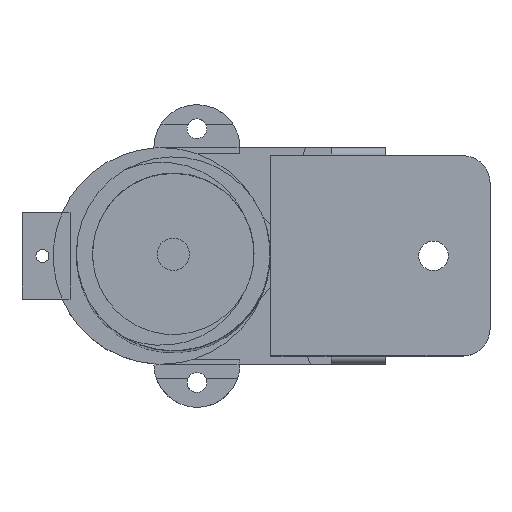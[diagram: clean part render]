
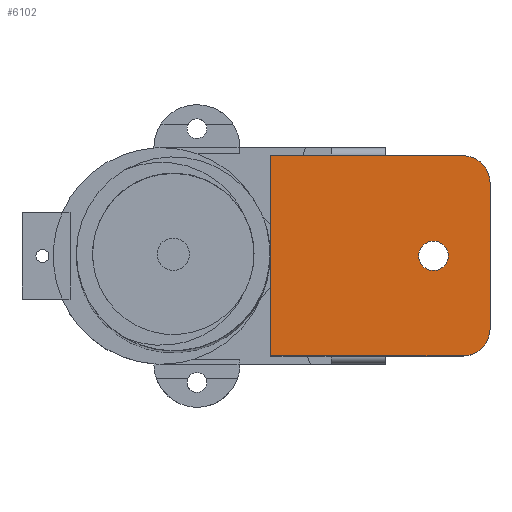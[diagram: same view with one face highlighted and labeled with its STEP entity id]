
A CAD part, top view. The second image highlights one B-rep face of the part: STEP entity #6102.
In plain terms, the highlighted planar face has unit normal (0, 0, 1).
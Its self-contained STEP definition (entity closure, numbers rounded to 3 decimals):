
#3898 = PLANE('',#3899);
#3899 = AXIS2_PLACEMENT_3D('',#3900,#3901,#3902);
#3900 = CARTESIAN_POINT('',(-27.612,18.6,22.6));
#3901 = DIRECTION('',(0.,1.,0.));
#3902 = DIRECTION('',(1.,0.,0.));
#4639 = PLANE('',#4640);
#4640 = AXIS2_PLACEMENT_3D('',#4641,#4642,#4643);
#4641 = CARTESIAN_POINT('',(13.137,-18.6,22.6));
#4642 = DIRECTION('',(0.,-1.,0.));
#4643 = DIRECTION('',(-1.,0.,0.));
#5168 = PLANE('',#5169);
#5169 = AXIS2_PLACEMENT_3D('',#5170,#5171,#5172);
#5170 = CARTESIAN_POINT('',(-27.612,-18.6,22.6));
#5171 = DIRECTION('',(-1.,0.,0.));
#5172 = DIRECTION('',(0.,1.,0.));
#5205 = EDGE_CURVE('',#5206,#5208,#5210,.T.);
#5206 = VERTEX_POINT('',#5207);
#5207 = CARTESIAN_POINT('',(-27.612,18.6,24.1));
#5208 = VERTEX_POINT('',#5209);
#5209 = CARTESIAN_POINT('',(8.137,18.6,24.1));
#5210 = SURFACE_CURVE('',#5211,(#5215,#5222),.PCURVE_S1.);
#5211 = LINE('',#5212,#5213);
#5212 = CARTESIAN_POINT('',(-27.612,18.6,24.1));
#5213 = VECTOR('',#5214,1.);
#5214 = DIRECTION('',(1.,0.,0.));
#5215 = PCURVE('',#3898,#5216);
#5216 = DEFINITIONAL_REPRESENTATION('',(#5217),#5221);
#5217 = LINE('',#5218,#5219);
#5218 = CARTESIAN_POINT('',(0.,-1.5));
#5219 = VECTOR('',#5220,1.);
#5220 = DIRECTION('',(1.,0.));
#5221 = ( GEOMETRIC_REPRESENTATION_CONTEXT(2) 
PARAMETRIC_REPRESENTATION_CONTEXT() REPRESENTATION_CONTEXT('2D SPACE',''
  ) );
#5222 = PCURVE('',#5223,#5228);
#5223 = PLANE('',#5224);
#5224 = AXIS2_PLACEMENT_3D('',#5225,#5226,#5227);
#5225 = CARTESIAN_POINT('',(-27.612,18.6,24.1));
#5226 = DIRECTION('',(0.,0.,1.));
#5227 = DIRECTION('',(1.,0.,0.));
#5228 = DEFINITIONAL_REPRESENTATION('',(#5229),#5233);
#5229 = LINE('',#5230,#5231);
#5230 = CARTESIAN_POINT('',(0.,0.));
#5231 = VECTOR('',#5232,1.);
#5232 = DIRECTION('',(1.,0.));
#5233 = ( GEOMETRIC_REPRESENTATION_CONTEXT(2) 
PARAMETRIC_REPRESENTATION_CONTEXT() REPRESENTATION_CONTEXT('2D SPACE',''
  ) );
#5251 = CYLINDRICAL_SURFACE('',#5252,5.);
#5252 = AXIS2_PLACEMENT_3D('',#5253,#5254,#5255);
#5253 = CARTESIAN_POINT('',(8.137,13.6,22.6));
#5254 = DIRECTION('',(0.,0.,1.));
#5255 = DIRECTION('',(1.,0.,0.));
#5709 = EDGE_CURVE('',#5710,#5712,#5714,.T.);
#5710 = VERTEX_POINT('',#5711);
#5711 = CARTESIAN_POINT('',(8.137,-18.6,24.1));
#5712 = VERTEX_POINT('',#5713);
#5713 = CARTESIAN_POINT('',(-27.612,-18.6,24.1));
#5714 = SURFACE_CURVE('',#5715,(#5719,#5726),.PCURVE_S1.);
#5715 = LINE('',#5716,#5717);
#5716 = CARTESIAN_POINT('',(13.137,-18.6,24.1));
#5717 = VECTOR('',#5718,1.);
#5718 = DIRECTION('',(-1.,0.,0.));
#5719 = PCURVE('',#4639,#5720);
#5720 = DEFINITIONAL_REPRESENTATION('',(#5721),#5725);
#5721 = LINE('',#5722,#5723);
#5722 = CARTESIAN_POINT('',(0.,-1.5));
#5723 = VECTOR('',#5724,1.);
#5724 = DIRECTION('',(1.,0.));
#5725 = ( GEOMETRIC_REPRESENTATION_CONTEXT(2) 
PARAMETRIC_REPRESENTATION_CONTEXT() REPRESENTATION_CONTEXT('2D SPACE',''
  ) );
#5726 = PCURVE('',#5223,#5727);
#5727 = DEFINITIONAL_REPRESENTATION('',(#5728),#5732);
#5728 = LINE('',#5729,#5730);
#5729 = CARTESIAN_POINT('',(40.749,-37.2));
#5730 = VECTOR('',#5731,1.);
#5731 = DIRECTION('',(-1.,0.));
#5732 = ( GEOMETRIC_REPRESENTATION_CONTEXT(2) 
PARAMETRIC_REPRESENTATION_CONTEXT() REPRESENTATION_CONTEXT('2D SPACE',''
  ) );
#5795 = CYLINDRICAL_SURFACE('',#5796,5.);
#5796 = AXIS2_PLACEMENT_3D('',#5797,#5798,#5799);
#5797 = CARTESIAN_POINT('',(8.137,-13.6,22.6));
#5798 = DIRECTION('',(0.,0.,1.));
#5799 = DIRECTION('',(1.,0.,0.));
#6080 = EDGE_CURVE('',#5712,#5206,#6081,.T.);
#6081 = SURFACE_CURVE('',#6082,(#6086,#6093),.PCURVE_S1.);
#6082 = LINE('',#6083,#6084);
#6083 = CARTESIAN_POINT('',(-27.612,-18.6,24.1));
#6084 = VECTOR('',#6085,1.);
#6085 = DIRECTION('',(0.,1.,0.));
#6086 = PCURVE('',#5168,#6087);
#6087 = DEFINITIONAL_REPRESENTATION('',(#6088),#6092);
#6088 = LINE('',#6089,#6090);
#6089 = CARTESIAN_POINT('',(0.,-1.5));
#6090 = VECTOR('',#6091,1.);
#6091 = DIRECTION('',(1.,0.));
#6092 = ( GEOMETRIC_REPRESENTATION_CONTEXT(2) 
PARAMETRIC_REPRESENTATION_CONTEXT() REPRESENTATION_CONTEXT('2D SPACE',''
  ) );
#6093 = PCURVE('',#5223,#6094);
#6094 = DEFINITIONAL_REPRESENTATION('',(#6095),#6099);
#6095 = LINE('',#6096,#6097);
#6096 = CARTESIAN_POINT('',(0.,-37.2));
#6097 = VECTOR('',#6098,1.);
#6098 = DIRECTION('',(0.,1.));
#6099 = ( GEOMETRIC_REPRESENTATION_CONTEXT(2) 
PARAMETRIC_REPRESENTATION_CONTEXT() REPRESENTATION_CONTEXT('2D SPACE',''
  ) );
#6102 = ADVANCED_FACE('',(#6103,#6186),#5223,.T.);
#6103 = FACE_BOUND('',#6104,.T.);
#6104 = EDGE_LOOP('',(#6105,#6135,#6157,#6158,#6159,#6160));
#6105 = ORIENTED_EDGE('',*,*,#6106,.F.);
#6106 = EDGE_CURVE('',#6107,#6109,#6111,.T.);
#6107 = VERTEX_POINT('',#6108);
#6108 = CARTESIAN_POINT('',(13.137,13.6,24.1));
#6109 = VERTEX_POINT('',#6110);
#6110 = CARTESIAN_POINT('',(13.137,-13.6,24.1));
#6111 = SURFACE_CURVE('',#6112,(#6116,#6123),.PCURVE_S1.);
#6112 = LINE('',#6113,#6114);
#6113 = CARTESIAN_POINT('',(13.137,18.6,24.1));
#6114 = VECTOR('',#6115,1.);
#6115 = DIRECTION('',(0.,-1.,0.));
#6116 = PCURVE('',#5223,#6117);
#6117 = DEFINITIONAL_REPRESENTATION('',(#6118),#6122);
#6118 = LINE('',#6119,#6120);
#6119 = CARTESIAN_POINT('',(40.749,0.));
#6120 = VECTOR('',#6121,1.);
#6121 = DIRECTION('',(0.,-1.));
#6122 = ( GEOMETRIC_REPRESENTATION_CONTEXT(2) 
PARAMETRIC_REPRESENTATION_CONTEXT() REPRESENTATION_CONTEXT('2D SPACE',''
  ) );
#6123 = PCURVE('',#6124,#6129);
#6124 = PLANE('',#6125);
#6125 = AXIS2_PLACEMENT_3D('',#6126,#6127,#6128);
#6126 = CARTESIAN_POINT('',(13.137,18.6,22.6));
#6127 = DIRECTION('',(1.,0.,0.));
#6128 = DIRECTION('',(0.,-1.,0.));
#6129 = DEFINITIONAL_REPRESENTATION('',(#6130),#6134);
#6130 = LINE('',#6131,#6132);
#6131 = CARTESIAN_POINT('',(0.,-1.5));
#6132 = VECTOR('',#6133,1.);
#6133 = DIRECTION('',(1.,0.));
#6134 = ( GEOMETRIC_REPRESENTATION_CONTEXT(2) 
PARAMETRIC_REPRESENTATION_CONTEXT() REPRESENTATION_CONTEXT('2D SPACE',''
  ) );
#6135 = ORIENTED_EDGE('',*,*,#6136,.T.);
#6136 = EDGE_CURVE('',#6107,#5208,#6137,.T.);
#6137 = SURFACE_CURVE('',#6138,(#6143,#6150),.PCURVE_S1.);
#6138 = CIRCLE('',#6139,5.);
#6139 = AXIS2_PLACEMENT_3D('',#6140,#6141,#6142);
#6140 = CARTESIAN_POINT('',(8.137,13.6,24.1));
#6141 = DIRECTION('',(0.,0.,1.));
#6142 = DIRECTION('',(0.,-1.,0.));
#6143 = PCURVE('',#5223,#6144);
#6144 = DEFINITIONAL_REPRESENTATION('',(#6145),#6149);
#6145 = CIRCLE('',#6146,5.);
#6146 = AXIS2_PLACEMENT_2D('',#6147,#6148);
#6147 = CARTESIAN_POINT('',(35.749,-5.));
#6148 = DIRECTION('',(0.,-1.));
#6149 = ( GEOMETRIC_REPRESENTATION_CONTEXT(2) 
PARAMETRIC_REPRESENTATION_CONTEXT() REPRESENTATION_CONTEXT('2D SPACE',''
  ) );
#6150 = PCURVE('',#5251,#6151);
#6151 = DEFINITIONAL_REPRESENTATION('',(#6152),#6156);
#6152 = LINE('',#6153,#6154);
#6153 = CARTESIAN_POINT('',(-1.571,1.5));
#6154 = VECTOR('',#6155,1.);
#6155 = DIRECTION('',(1.,0.));
#6156 = ( GEOMETRIC_REPRESENTATION_CONTEXT(2) 
PARAMETRIC_REPRESENTATION_CONTEXT() REPRESENTATION_CONTEXT('2D SPACE',''
  ) );
#6157 = ORIENTED_EDGE('',*,*,#5205,.F.);
#6158 = ORIENTED_EDGE('',*,*,#6080,.F.);
#6159 = ORIENTED_EDGE('',*,*,#5709,.F.);
#6160 = ORIENTED_EDGE('',*,*,#6161,.F.);
#6161 = EDGE_CURVE('',#6109,#5710,#6162,.T.);
#6162 = SURFACE_CURVE('',#6163,(#6168,#6179),.PCURVE_S1.);
#6163 = CIRCLE('',#6164,5.);
#6164 = AXIS2_PLACEMENT_3D('',#6165,#6166,#6167);
#6165 = CARTESIAN_POINT('',(8.137,-13.6,24.1));
#6166 = DIRECTION('',(0.,0.,-1.));
#6167 = DIRECTION('',(0.,-1.,0.));
#6168 = PCURVE('',#5223,#6169);
#6169 = DEFINITIONAL_REPRESENTATION('',(#6170),#6178);
#6170 = ( BOUNDED_CURVE() B_SPLINE_CURVE(2,(#6171,#6172,#6173,#6174,
#6175,#6176,#6177),.UNSPECIFIED.,.T.,.F.) B_SPLINE_CURVE_WITH_KNOTS((1,2
    ,2,2,2,1),(-2.094,0.,2.094,4.189,
6.283,8.378),.UNSPECIFIED.) CURVE() 
GEOMETRIC_REPRESENTATION_ITEM() RATIONAL_B_SPLINE_CURVE((1.,0.5,1.,0.5,
1.,0.5,1.)) REPRESENTATION_ITEM('') );
#6171 = CARTESIAN_POINT('',(35.749,-37.2));
#6172 = CARTESIAN_POINT('',(27.089,-37.2));
#6173 = CARTESIAN_POINT('',(31.419,-29.7));
#6174 = CARTESIAN_POINT('',(35.749,-22.2));
#6175 = CARTESIAN_POINT('',(40.079,-29.7));
#6176 = CARTESIAN_POINT('',(44.409,-37.2));
#6177 = CARTESIAN_POINT('',(35.749,-37.2));
#6178 = ( GEOMETRIC_REPRESENTATION_CONTEXT(2) 
PARAMETRIC_REPRESENTATION_CONTEXT() REPRESENTATION_CONTEXT('2D SPACE',''
  ) );
#6179 = PCURVE('',#5795,#6180);
#6180 = DEFINITIONAL_REPRESENTATION('',(#6181),#6185);
#6181 = LINE('',#6182,#6183);
#6182 = CARTESIAN_POINT('',(4.712,1.5));
#6183 = VECTOR('',#6184,1.);
#6184 = DIRECTION('',(-1.,0.));
#6185 = ( GEOMETRIC_REPRESENTATION_CONTEXT(2) 
PARAMETRIC_REPRESENTATION_CONTEXT() REPRESENTATION_CONTEXT('2D SPACE',''
  ) );
#6186 = FACE_BOUND('',#6187,.T.);
#6187 = EDGE_LOOP('',(#6188));
#6188 = ORIENTED_EDGE('',*,*,#6189,.T.);
#6189 = EDGE_CURVE('',#6190,#6190,#6192,.T.);
#6190 = VERTEX_POINT('',#6191);
#6191 = CARTESIAN_POINT('',(5.387,0.,24.1));
#6192 = SURFACE_CURVE('',#6193,(#6198,#6209),.PCURVE_S1.);
#6193 = CIRCLE('',#6194,2.75);
#6194 = AXIS2_PLACEMENT_3D('',#6195,#6196,#6197);
#6195 = CARTESIAN_POINT('',(2.637,0.,24.1));
#6196 = DIRECTION('',(0.,0.,-1.));
#6197 = DIRECTION('',(1.,0.,0.));
#6198 = PCURVE('',#5223,#6199);
#6199 = DEFINITIONAL_REPRESENTATION('',(#6200),#6208);
#6200 = ( BOUNDED_CURVE() B_SPLINE_CURVE(2,(#6201,#6202,#6203,#6204,
#6205,#6206,#6207),.UNSPECIFIED.,.F.,.F.) B_SPLINE_CURVE_WITH_KNOTS((1,2
    ,2,2,2,1),(-2.094,0.,2.094,4.189,
6.283,8.378),.UNSPECIFIED.) CURVE() 
GEOMETRIC_REPRESENTATION_ITEM() RATIONAL_B_SPLINE_CURVE((1.,0.5,1.,0.5,
1.,0.5,1.)) REPRESENTATION_ITEM('') );
#6201 = CARTESIAN_POINT('',(32.999,-18.6));
#6202 = CARTESIAN_POINT('',(32.999,-23.363));
#6203 = CARTESIAN_POINT('',(28.874,-20.982));
#6204 = CARTESIAN_POINT('',(24.749,-18.6));
#6205 = CARTESIAN_POINT('',(28.874,-16.218));
#6206 = CARTESIAN_POINT('',(32.999,-13.837));
#6207 = CARTESIAN_POINT('',(32.999,-18.6));
#6208 = ( GEOMETRIC_REPRESENTATION_CONTEXT(2) 
PARAMETRIC_REPRESENTATION_CONTEXT() REPRESENTATION_CONTEXT('2D SPACE',''
  ) );
#6209 = PCURVE('',#6210,#6215);
#6210 = CYLINDRICAL_SURFACE('',#6211,2.75);
#6211 = AXIS2_PLACEMENT_3D('',#6212,#6213,#6214);
#6212 = CARTESIAN_POINT('',(2.637,0.,0.));
#6213 = DIRECTION('',(0.,0.,-1.));
#6214 = DIRECTION('',(1.,0.,0.));
#6215 = DEFINITIONAL_REPRESENTATION('',(#6216),#6220);
#6216 = LINE('',#6217,#6218);
#6217 = CARTESIAN_POINT('',(0.,-24.1));
#6218 = VECTOR('',#6219,1.);
#6219 = DIRECTION('',(1.,0.));
#6220 = ( GEOMETRIC_REPRESENTATION_CONTEXT(2) 
PARAMETRIC_REPRESENTATION_CONTEXT() REPRESENTATION_CONTEXT('2D SPACE',''
  ) );
